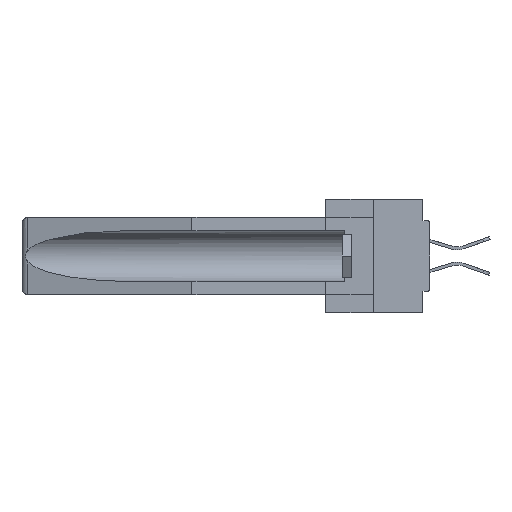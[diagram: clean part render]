
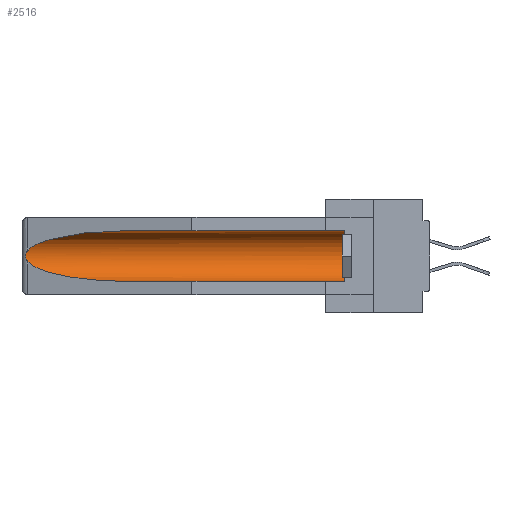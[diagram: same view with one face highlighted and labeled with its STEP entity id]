
A CAD part, left-side view. The second image highlights one B-rep face of the part: STEP entity #2516.
In plain terms, the highlighted cylindrical face has radius 2.857 mm (diameter 5.715 mm), a partial arc.
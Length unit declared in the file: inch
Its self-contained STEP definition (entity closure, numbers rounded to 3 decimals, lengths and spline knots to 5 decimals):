
#111 = CARTESIAN_POINT ( 'NONE',  ( 0.26537, 1.52718, -0.19328 ) ) ;
#499 =( BOUNDED_CURVE ( )  B_SPLINE_CURVE ( 3, ( #11311, #30103, #24694, #3266 ),
 .UNSPECIFIED., .F., .F. ) 
 B_SPLINE_CURVE_WITH_KNOTS ( ( 4, 4 ),
 ( 0.1948, 1.5708 ),
 .UNSPECIFIED. ) 
 CURVE ( )  GEOMETRIC_REPRESENTATION_ITEM ( )  RATIONAL_B_SPLINE_CURVE ( ( 1., 0.848, 0.848, 1. ) ) 
 REPRESENTATION_ITEM ( '' )  );
#643 = CARTESIAN_POINT ( 'NONE',  ( 0.155, 0.126, -0.1715 ) ) ;
#1189 = CARTESIAN_POINT ( 'NONE',  ( 0.26655, 1.53094, -0.18657 ) ) ;
#2075 = DIRECTION ( 'NONE',  ( 0., 1., 0. ) ) ;
#2380 = EDGE_CURVE ( 'NONE', #17182, #10672, #15742, .T. ) ;
#2516 = ADVANCED_FACE ( 'NONE', ( #25505 ), #17045, .F. ) ;
#3156 = VERTEX_POINT ( 'NONE', #21662 ) ;
#3266 = CARTESIAN_POINT ( 'NONE',  ( 0.155, 1.07973, -0.284 ) ) ;
#3794 = CARTESIAN_POINT ( 'NONE',  ( 0.2675, 1.53308, -0.17534 ) ) ;
#4725 = EDGE_CURVE ( 'NONE', #23797, #3156, #14165, .T. ) ;
#4850 = CARTESIAN_POINT ( 'NONE',  ( 0.155, -0.30754, -0.284 ) ) ;
#5538 = EDGE_CURVE ( 'NONE', #3156, #19941, #18933, .T. ) ;
#6098 = DIRECTION ( 'NONE',  ( 0., 1., 0. ) ) ;
#6497 = ORIENTED_EDGE ( 'NONE', *, *, #25619, .T. ) ;
#6888 = ORIENTED_EDGE ( 'NONE', *, *, #5538, .T. ) ;
#7180 = CARTESIAN_POINT ( 'NONE',  ( 0.21114, 1.30732, -0.059 ) ) ;
#7518 = VECTOR ( 'NONE', #2075, 39.37008 ) ;
#9324 = VERTEX_POINT ( 'NONE', #11908 ) ;
#10672 = VERTEX_POINT ( 'NONE', #17258 ) ;
#11311 = CARTESIAN_POINT ( 'NONE',  ( 0.26537, 1.52718, -0.19328 ) ) ;
#11401 = DIRECTION ( 'NONE',  ( 0., -1., 0. ) ) ;
#11908 = CARTESIAN_POINT ( 'NONE',  ( 0.155, 1.07973, -0.284 ) ) ;
#12651 = EDGE_CURVE ( 'NONE', #17182, #9324, #13584, .T. ) ;
#12731 = CARTESIAN_POINT ( 'NONE',  ( 0.155, 1.07973, -0.059 ) ) ;
#13584 = LINE ( 'NONE', #4850, #16956 ) ;
#14165 =( BOUNDED_CURVE ( )  B_SPLINE_CURVE ( 3, ( #12731, #7180, #28689, #31765 ),
 .UNSPECIFIED., .F., .T. ) 
 B_SPLINE_CURVE_WITH_KNOTS ( ( 4, 4 ),
 ( 4.71239, 6.08839 ),
 .UNSPECIFIED. ) 
 CURVE ( )  GEOMETRIC_REPRESENTATION_ITEM ( )  RATIONAL_B_SPLINE_CURVE ( ( 1., 0.848, 0.848, 1. ) ) 
 REPRESENTATION_ITEM ( '' )  );
#14504 = EDGE_CURVE ( 'NONE', #10672, #23797, #32511, .T. ) ;
#15742 = CIRCLE ( 'NONE', #32929, 0.1125 ) ;
#16956 = VECTOR ( 'NONE', #26254, 39.37008 ) ;
#17045 = CYLINDRICAL_SURFACE ( 'NONE', #33396, 0.1125 ) ;
#17182 = VERTEX_POINT ( 'NONE', #34887 ) ;
#17258 = CARTESIAN_POINT ( 'NONE',  ( 0.155, 0.126, -0.059 ) ) ;
#17383 = CARTESIAN_POINT ( 'NONE',  ( 0.26537, 1.52718, -0.14972 ) ) ;
#17506 = CARTESIAN_POINT ( 'NONE',  ( 0.26597, 1.5296, -0.19026 ) ) ;
#18933 = B_SPLINE_CURVE_WITH_KNOTS ( 'NONE', 3,
 ( #17383, #19873, #33744, #25680, #33278, #3794, #30742, #1189, #17506, #20115 ),
 .UNSPECIFIED., .F., .F.,
 ( 4, 2, 2, 2, 4 ),
 ( 0., 0.00029, 0.00058, 0.00087, 0.00117 ),
 .UNSPECIFIED. ) ;
#19873 = CARTESIAN_POINT ( 'NONE',  ( 0.26597, 1.52961, -0.15275 ) ) ;
#19941 = VERTEX_POINT ( 'NONE', #111 ) ;
#20115 = CARTESIAN_POINT ( 'NONE',  ( 0.26537, 1.52718, -0.19328 ) ) ;
#21559 = ORIENTED_EDGE ( 'NONE', *, *, #2380, .T. ) ;
#21662 = CARTESIAN_POINT ( 'NONE',  ( 0.26537, 1.52718, -0.14972 ) ) ;
#23248 = ORIENTED_EDGE ( 'NONE', *, *, #12651, .F. ) ;
#23327 = DIRECTION ( 'NONE',  ( 0., 0., 1. ) ) ;
#23797 = VERTEX_POINT ( 'NONE', #30040 ) ;
#24694 = CARTESIAN_POINT ( 'NONE',  ( 0.21114, 1.30732, -0.284 ) ) ;
#25505 = FACE_OUTER_BOUND ( 'NONE', #30022, .T. ) ;
#25619 = EDGE_CURVE ( 'NONE', #19941, #9324, #499, .T. ) ;
#25680 = CARTESIAN_POINT ( 'NONE',  ( 0.2673, 1.5327, -0.16383 ) ) ;
#26148 = ORIENTED_EDGE ( 'NONE', *, *, #4725, .T. ) ;
#26254 = DIRECTION ( 'NONE',  ( 0., 1., 0. ) ) ;
#27737 = DIRECTION ( 'NONE',  ( 0., 0., 1. ) ) ;
#28017 = ORIENTED_EDGE ( 'NONE', *, *, #14504, .T. ) ;
#28689 = CARTESIAN_POINT ( 'NONE',  ( 0.25451, 1.48313, -0.09465 ) ) ;
#30022 = EDGE_LOOP ( 'NONE', ( #26148, #6888, #6497, #23248, #21559, #28017 ) ) ;
#30040 = CARTESIAN_POINT ( 'NONE',  ( 0.155, 1.07973, -0.059 ) ) ;
#30103 = CARTESIAN_POINT ( 'NONE',  ( 0.25451, 1.48313, -0.24835 ) ) ;
#30311 = CARTESIAN_POINT ( 'NONE',  ( 0.155, -0.30754, -0.1715 ) ) ;
#30742 = CARTESIAN_POINT ( 'NONE',  ( 0.2673, 1.53269, -0.17917 ) ) ;
#31765 = CARTESIAN_POINT ( 'NONE',  ( 0.26537, 1.52718, -0.14972 ) ) ;
#32511 = LINE ( 'NONE', #34653, #7518 ) ;
#32929 = AXIS2_PLACEMENT_3D ( 'NONE', #643, #11401, #27737 ) ;
#33278 = CARTESIAN_POINT ( 'NONE',  ( 0.2675, 1.53308, -0.16763 ) ) ;
#33396 = AXIS2_PLACEMENT_3D ( 'NONE', #30311, #6098, #23327 ) ;
#33744 = CARTESIAN_POINT ( 'NONE',  ( 0.26654, 1.53092, -0.15636 ) ) ;
#34653 = CARTESIAN_POINT ( 'NONE',  ( 0.155, -0.30754, -0.059 ) ) ;
#34887 = CARTESIAN_POINT ( 'NONE',  ( 0.155, 0.126, -0.284 ) ) ;
